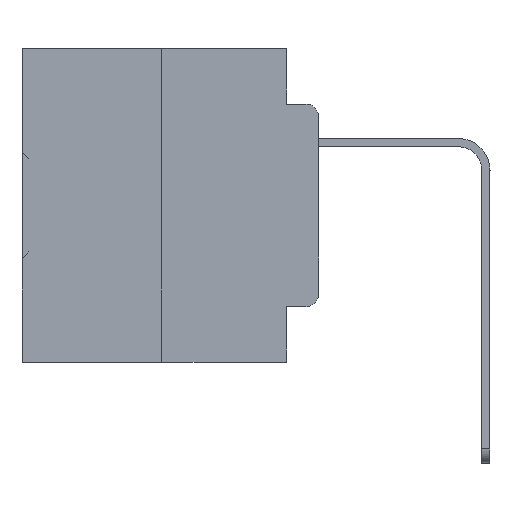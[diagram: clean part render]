
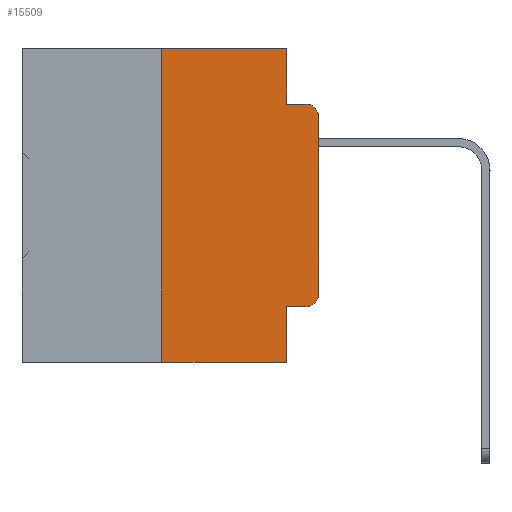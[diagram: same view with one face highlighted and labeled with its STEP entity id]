
A CAD part, left-side view. The second image highlights one B-rep face of the part: STEP entity #15509.
In plain terms, the highlighted planar face has unit normal (-1, 0, 0).
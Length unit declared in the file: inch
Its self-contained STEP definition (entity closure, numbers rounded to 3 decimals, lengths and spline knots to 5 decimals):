
#125 = VECTOR ( 'NONE', #23417, 39.37008 ) ;
#405 = DIRECTION ( 'NONE',  ( 1., 0., 0. ) ) ;
#1089 = CARTESIAN_POINT ( 'NONE',  ( 0., 0.051, 0. ) ) ;
#1866 = AXIS2_PLACEMENT_3D ( 'NONE', #34008, #405, #14398 ) ;
#2878 = DIRECTION ( 'NONE',  ( 0., 0., -1. ) ) ;
#3690 = VERTEX_POINT ( 'NONE', #11384 ) ;
#3827 = FACE_OUTER_BOUND ( 'NONE', #18196, .T. ) ;
#4939 = LINE ( 'NONE', #12540, #33708 ) ;
#5364 = ORIENTED_EDGE ( 'NONE', *, *, #13908, .T. ) ;
#5436 = DIRECTION ( 'NONE',  ( 0., 0., -1. ) ) ;
#6148 = PLANE ( 'NONE',  #1866 ) ;
#6494 = DIRECTION ( 'NONE',  ( 0., 0., 1. ) ) ;
#8080 = LINE ( 'NONE', #1089, #29854 ) ;
#8196 = CARTESIAN_POINT ( 'NONE',  ( 0., 0.25, -0.5 ) ) ;
#8253 = AXIS2_PLACEMENT_3D ( 'NONE', #22086, #24869, #5436 ) ;
#9020 = AXIS2_PLACEMENT_3D ( 'NONE', #10811, #27332, #35755 ) ;
#9210 = DIRECTION ( 'NONE',  ( 0., 0., 1. ) ) ;
#9572 = VERTEX_POINT ( 'NONE', #24782 ) ;
#10018 = CARTESIAN_POINT ( 'NONE',  ( 0., 0., -0.3915 ) ) ;
#10476 = ORIENTED_EDGE ( 'NONE', *, *, #34265, .T. ) ;
#10565 = DIRECTION ( 'NONE',  ( 0., -1., 0. ) ) ;
#10811 = CARTESIAN_POINT ( 'NONE',  ( 0., 0.02, -0.1085 ) ) ;
#11347 = ORIENTED_EDGE ( 'NONE', *, *, #32355, .T. ) ;
#11384 = CARTESIAN_POINT ( 'NONE',  ( 0., 0.051, -0.0885 ) ) ;
#11848 = VERTEX_POINT ( 'NONE', #8196 ) ;
#12540 = CARTESIAN_POINT ( 'NONE',  ( 0., 0.473, 0. ) ) ;
#12642 = ORIENTED_EDGE ( 'NONE', *, *, #14777, .F. ) ;
#12893 = EDGE_CURVE ( 'NONE', #3690, #21525, #14484, .T. ) ;
#13052 = EDGE_CURVE ( 'NONE', #11848, #31564, #14026, .T. ) ;
#13281 = LINE ( 'NONE', #25467, #27185 ) ;
#13738 = VECTOR ( 'NONE', #6494, 39.37008 ) ;
#13908 = EDGE_CURVE ( 'NONE', #25369, #23623, #30084, .T. ) ;
#14026 = LINE ( 'NONE', #35374, #24023 ) ;
#14185 = ORIENTED_EDGE ( 'NONE', *, *, #29069, .T. ) ;
#14398 = DIRECTION ( 'NONE',  ( 0., 0., -1. ) ) ;
#14484 = LINE ( 'NONE', #20505, #125 ) ;
#14500 = CARTESIAN_POINT ( 'NONE',  ( 0., 0.25, 0. ) ) ;
#14777 = EDGE_CURVE ( 'NONE', #9572, #3690, #31740, .T. ) ;
#15266 = VECTOR ( 'NONE', #15956, 39.37008 ) ;
#15509 = ADVANCED_FACE ( 'NONE', ( #3827 ), #6148, .F. ) ;
#15956 = DIRECTION ( 'NONE',  ( 0., -1., 0. ) ) ;
#16278 = ORIENTED_EDGE ( 'NONE', *, *, #35335, .F. ) ;
#17604 = CARTESIAN_POINT ( 'NONE',  ( 0., 0.051, -0.4115 ) ) ;
#18196 = EDGE_LOOP ( 'NONE', ( #14185, #10476, #23100, #12642, #16278, #27433, #18801, #30838, #5364, #11347 ) ) ;
#18801 = ORIENTED_EDGE ( 'NONE', *, *, #13052, .T. ) ;
#20505 = CARTESIAN_POINT ( 'NONE',  ( 0., 0.051, -0.0885 ) ) ;
#21113 = LINE ( 'NONE', #14500, #13738 ) ;
#21525 = VERTEX_POINT ( 'NONE', #28590 ) ;
#21614 = EDGE_CURVE ( 'NONE', #25369, #31564, #8080, .T. ) ;
#21998 = CIRCLE ( 'NONE', #9020, 0.02 ) ;
#22072 = EDGE_CURVE ( 'NONE', #11848, #22904, #21113, .T. ) ;
#22086 = CARTESIAN_POINT ( 'NONE',  ( 0., 0.02, -0.3915 ) ) ;
#22904 = VERTEX_POINT ( 'NONE', #36007 ) ;
#23100 = ORIENTED_EDGE ( 'NONE', *, *, #12893, .F. ) ;
#23417 = DIRECTION ( 'NONE',  ( 0., -1., 0. ) ) ;
#23623 = VERTEX_POINT ( 'NONE', #24950 ) ;
#24023 = VECTOR ( 'NONE', #10565, 39.37008 ) ;
#24304 = VECTOR ( 'NONE', #2878, 39.37008 ) ;
#24782 = CARTESIAN_POINT ( 'NONE',  ( 0., 0.051, 0. ) ) ;
#24869 = DIRECTION ( 'NONE',  ( -1., 0., 0. ) ) ;
#24950 = CARTESIAN_POINT ( 'NONE',  ( 0., 0.02, -0.4115 ) ) ;
#25369 = VERTEX_POINT ( 'NONE', #17604 ) ;
#25467 = CARTESIAN_POINT ( 'NONE',  ( 0., 0., 0. ) ) ;
#25613 = CARTESIAN_POINT ( 'NONE',  ( 0., 0.051, 0. ) ) ;
#26003 = CIRCLE ( 'NONE', #8253, 0.02 ) ;
#27185 = VECTOR ( 'NONE', #9210, 39.37008 ) ;
#27332 = DIRECTION ( 'NONE',  ( -1., 0., 0. ) ) ;
#27433 = ORIENTED_EDGE ( 'NONE', *, *, #22072, .F. ) ;
#27737 = VERTEX_POINT ( 'NONE', #10018 ) ;
#28590 = CARTESIAN_POINT ( 'NONE',  ( 0., 0.02, -0.0885 ) ) ;
#28710 = VERTEX_POINT ( 'NONE', #34782 ) ;
#29069 = EDGE_CURVE ( 'NONE', #27737, #28710, #13281, .T. ) ;
#29854 = VECTOR ( 'NONE', #34557, 39.37008 ) ;
#30084 = LINE ( 'NONE', #32409, #15266 ) ;
#30838 = ORIENTED_EDGE ( 'NONE', *, *, #21614, .F. ) ;
#31564 = VERTEX_POINT ( 'NONE', #35686 ) ;
#31740 = LINE ( 'NONE', #25613, #24304 ) ;
#31751 = DIRECTION ( 'NONE',  ( 0., -1., 0. ) ) ;
#32355 = EDGE_CURVE ( 'NONE', #23623, #27737, #26003, .T. ) ;
#32409 = CARTESIAN_POINT ( 'NONE',  ( 0., 0.051, -0.4115 ) ) ;
#33708 = VECTOR ( 'NONE', #31751, 39.37008 ) ;
#34008 = CARTESIAN_POINT ( 'NONE',  ( 0., 0.473, 0. ) ) ;
#34265 = EDGE_CURVE ( 'NONE', #28710, #21525, #21998, .T. ) ;
#34557 = DIRECTION ( 'NONE',  ( 0., 0., -1. ) ) ;
#34782 = CARTESIAN_POINT ( 'NONE',  ( 0., 0., -0.1085 ) ) ;
#35335 = EDGE_CURVE ( 'NONE', #22904, #9572, #4939, .T. ) ;
#35374 = CARTESIAN_POINT ( 'NONE',  ( 0., 0.473, -0.5 ) ) ;
#35686 = CARTESIAN_POINT ( 'NONE',  ( 0., 0.051, -0.5 ) ) ;
#35755 = DIRECTION ( 'NONE',  ( 0., 0., -1. ) ) ;
#36007 = CARTESIAN_POINT ( 'NONE',  ( 0., 0.25, 0. ) ) ;
